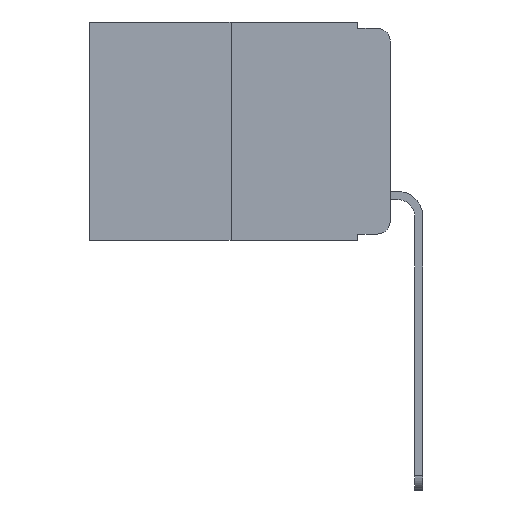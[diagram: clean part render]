
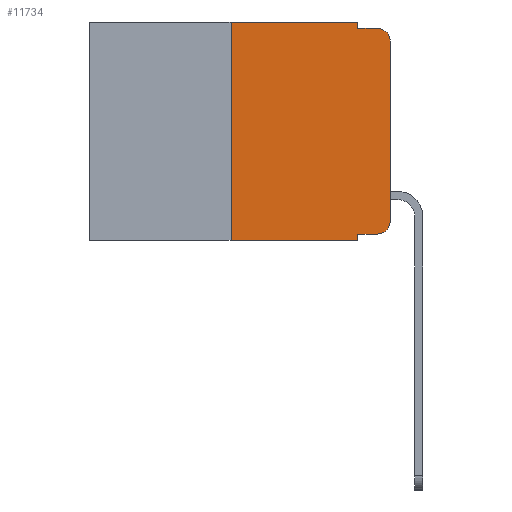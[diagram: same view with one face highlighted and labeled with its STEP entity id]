
A CAD part, left-side view. The second image highlights one B-rep face of the part: STEP entity #11734.
In plain terms, the highlighted planar face has unit normal (-1, 0, 0).
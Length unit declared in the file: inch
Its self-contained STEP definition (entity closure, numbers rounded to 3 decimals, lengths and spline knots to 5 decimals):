
#814 = DIRECTION ( 'NONE',  ( 1., 0., 0. ) ) ;
#1221 = VECTOR ( 'NONE', #9733, 39.37008 ) ;
#1255 = ORIENTED_EDGE ( 'NONE', *, *, #12647, .T. ) ;
#1316 = EDGE_CURVE ( 'NONE', #5312, #3000, #2925, .T. ) ;
#1612 = VECTOR ( 'NONE', #14065, 39.37008 ) ;
#1736 = CARTESIAN_POINT ( 'NONE',  ( 0., 0.051, -0.343 ) ) ;
#1845 = VECTOR ( 'NONE', #5614, 39.37008 ) ;
#2032 = PLANE ( 'NONE',  #2866 ) ;
#2044 = DIRECTION ( 'NONE',  ( 0., -1., 0. ) ) ;
#2140 = DIRECTION ( 'NONE',  ( 0., 0., 1. ) ) ;
#2213 = CARTESIAN_POINT ( 'NONE',  ( 0., 0.02, -0.01 ) ) ;
#2382 = EDGE_CURVE ( 'NONE', #12240, #8112, #5388, .T. ) ;
#2521 = DIRECTION ( 'NONE',  ( -1., 0., 0. ) ) ;
#2849 = LINE ( 'NONE', #9254, #7954 ) ;
#2866 = AXIS2_PLACEMENT_3D ( 'NONE', #13320, #814, #13231 ) ;
#2925 = CIRCLE ( 'NONE', #11322, 0.02 ) ;
#3000 = VERTEX_POINT ( 'NONE', #13026 ) ;
#3025 = CARTESIAN_POINT ( 'NONE',  ( 0., 0.473, -0.343 ) ) ;
#3796 = CARTESIAN_POINT ( 'NONE',  ( 0., 0.051, 0. ) ) ;
#4057 = CARTESIAN_POINT ( 'NONE',  ( 0., 0.051, 0. ) ) ;
#4080 = CARTESIAN_POINT ( 'NONE',  ( 0., 0.02, -0.313 ) ) ;
#4366 = CARTESIAN_POINT ( 'NONE',  ( 0., 0.051, -0.01 ) ) ;
#4404 = CARTESIAN_POINT ( 'NONE',  ( 0., 0., -0.03 ) ) ;
#4551 = CARTESIAN_POINT ( 'NONE',  ( 0., 0.25, 0. ) ) ;
#4824 = DIRECTION ( 'NONE',  ( 0., -1., 0. ) ) ;
#5212 = CARTESIAN_POINT ( 'NONE',  ( 0., 0.25, 0. ) ) ;
#5234 = EDGE_CURVE ( 'NONE', #11900, #9320, #8073, .T. ) ;
#5312 = VERTEX_POINT ( 'NONE', #7989 ) ;
#5334 = EDGE_CURVE ( 'NONE', #11943, #14444, #9328, .T. ) ;
#5338 = FACE_OUTER_BOUND ( 'NONE', #6429, .T. ) ;
#5388 = LINE ( 'NONE', #3796, #12662 ) ;
#5554 = CARTESIAN_POINT ( 'NONE',  ( 0., 0.473, 0. ) ) ;
#5614 = DIRECTION ( 'NONE',  ( 0., -1., 0. ) ) ;
#6429 = EDGE_LOOP ( 'NONE', ( #1255, #8812, #9534, #10613, #12737, #11394, #9628, #10872, #11694, #12774 ) ) ;
#6497 = CARTESIAN_POINT ( 'NONE',  ( 0., 0., 0. ) ) ;
#6517 = EDGE_CURVE ( 'NONE', #9320, #14255, #13662, .T. ) ;
#7268 = LINE ( 'NONE', #6497, #13465 ) ;
#7452 = DIRECTION ( 'NONE',  ( 0., 0., -1. ) ) ;
#7564 = EDGE_CURVE ( 'NONE', #14255, #11294, #13387, .T. ) ;
#7954 = VECTOR ( 'NONE', #4824, 39.37008 ) ;
#7989 = CARTESIAN_POINT ( 'NONE',  ( 0., 0.02, -0.333 ) ) ;
#8035 = CARTESIAN_POINT ( 'NONE',  ( 0., 0.02, -0.03 ) ) ;
#8073 = LINE ( 'NONE', #4551, #10933 ) ;
#8112 = VERTEX_POINT ( 'NONE', #1736 ) ;
#8137 = EDGE_CURVE ( 'NONE', #11900, #8112, #10109, .T. ) ;
#8792 = DIRECTION ( 'NONE',  ( 0., 0., 1. ) ) ;
#8812 = ORIENTED_EDGE ( 'NONE', *, *, #5334, .T. ) ;
#8835 = CARTESIAN_POINT ( 'NONE',  ( 0., 0.051, 0. ) ) ;
#9254 = CARTESIAN_POINT ( 'NONE',  ( 0., 0.051, -0.333 ) ) ;
#9320 = VERTEX_POINT ( 'NONE', #5212 ) ;
#9328 = CIRCLE ( 'NONE', #12364, 0.02 ) ;
#9534 = ORIENTED_EDGE ( 'NONE', *, *, #13299, .F. ) ;
#9536 = DIRECTION ( 'NONE',  ( 0., 0., -1. ) ) ;
#9628 = ORIENTED_EDGE ( 'NONE', *, *, #8137, .T. ) ;
#9733 = DIRECTION ( 'NONE',  ( 0., 0., -1. ) ) ;
#9948 = LINE ( 'NONE', #13335, #12406 ) ;
#10049 = CARTESIAN_POINT ( 'NONE',  ( 0., 0.25, -0.343 ) ) ;
#10109 = LINE ( 'NONE', #3025, #1612 ) ;
#10613 = ORIENTED_EDGE ( 'NONE', *, *, #7564, .F. ) ;
#10872 = ORIENTED_EDGE ( 'NONE', *, *, #2382, .F. ) ;
#10933 = VECTOR ( 'NONE', #2140, 39.37008 ) ;
#11294 = VERTEX_POINT ( 'NONE', #4366 ) ;
#11322 = AXIS2_PLACEMENT_3D ( 'NONE', #4080, #14192, #7452 ) ;
#11394 = ORIENTED_EDGE ( 'NONE', *, *, #5234, .F. ) ;
#11694 = ORIENTED_EDGE ( 'NONE', *, *, #13851, .T. ) ;
#11734 = ADVANCED_FACE ( 'NONE', ( #5338 ), #2032, .F. ) ;
#11900 = VERTEX_POINT ( 'NONE', #10049 ) ;
#11943 = VERTEX_POINT ( 'NONE', #4404 ) ;
#12240 = VERTEX_POINT ( 'NONE', #13702 ) ;
#12364 = AXIS2_PLACEMENT_3D ( 'NONE', #8035, #2521, #13752 ) ;
#12406 = VECTOR ( 'NONE', #2044, 39.37008 ) ;
#12647 = EDGE_CURVE ( 'NONE', #3000, #11943, #7268, .T. ) ;
#12662 = VECTOR ( 'NONE', #9536, 39.37008 ) ;
#12737 = ORIENTED_EDGE ( 'NONE', *, *, #6517, .F. ) ;
#12774 = ORIENTED_EDGE ( 'NONE', *, *, #1316, .T. ) ;
#13026 = CARTESIAN_POINT ( 'NONE',  ( 0., 0., -0.313 ) ) ;
#13231 = DIRECTION ( 'NONE',  ( 0., 0., -1. ) ) ;
#13299 = EDGE_CURVE ( 'NONE', #11294, #14444, #9948, .T. ) ;
#13320 = CARTESIAN_POINT ( 'NONE',  ( 0., 0.473, 0. ) ) ;
#13335 = CARTESIAN_POINT ( 'NONE',  ( 0., 0.051, -0.01 ) ) ;
#13387 = LINE ( 'NONE', #8835, #1221 ) ;
#13465 = VECTOR ( 'NONE', #8792, 39.37008 ) ;
#13662 = LINE ( 'NONE', #5554, #1845 ) ;
#13702 = CARTESIAN_POINT ( 'NONE',  ( 0., 0.051, -0.333 ) ) ;
#13752 = DIRECTION ( 'NONE',  ( 0., 0., -1. ) ) ;
#13851 = EDGE_CURVE ( 'NONE', #12240, #5312, #2849, .T. ) ;
#14065 = DIRECTION ( 'NONE',  ( 0., -1., 0. ) ) ;
#14192 = DIRECTION ( 'NONE',  ( -1., 0., 0. ) ) ;
#14255 = VERTEX_POINT ( 'NONE', #4057 ) ;
#14444 = VERTEX_POINT ( 'NONE', #2213 ) ;
